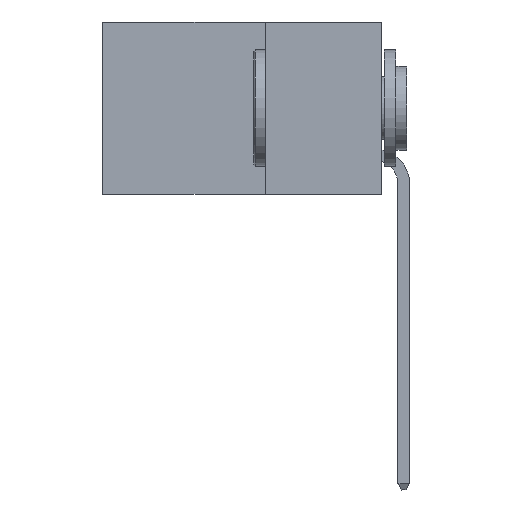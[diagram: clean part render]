
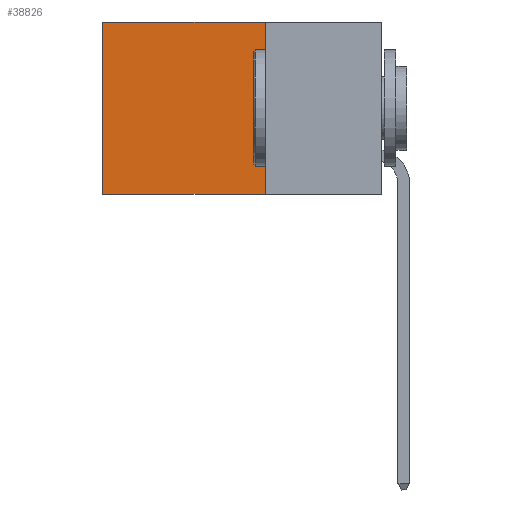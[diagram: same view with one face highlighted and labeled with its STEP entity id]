
A CAD part, left-side view. The second image highlights one B-rep face of the part: STEP entity #38826.
In plain terms, the highlighted planar face has unit normal (-1, 0, 0).
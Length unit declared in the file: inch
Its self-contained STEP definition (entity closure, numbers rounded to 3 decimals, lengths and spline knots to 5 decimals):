
#801 = LINE ( 'NONE', #12508, #32466 ) ;
#862 = LINE ( 'NONE', #8321, #16173 ) ;
#1087 = EDGE_CURVE ( 'NONE', #3247, #13767, #862, .T. ) ;
#1988 = EDGE_CURVE ( 'NONE', #23675, #22558, #22337, .T. ) ;
#3247 = VERTEX_POINT ( 'NONE', #31395 ) ;
#3289 = DIRECTION ( 'NONE',  ( 0., 0., -1. ) ) ;
#5727 = AXIS2_PLACEMENT_3D ( 'NONE', #35672, #17251, #38776 ) ;
#6565 = VECTOR ( 'NONE', #39519, 39.37008 ) ;
#8321 = CARTESIAN_POINT ( 'NONE',  ( 0.2875, 0.25, 0. ) ) ;
#8810 = CARTESIAN_POINT ( 'NONE',  ( 0.2875, 0.25, 0. ) ) ;
#12508 = CARTESIAN_POINT ( 'NONE',  ( 0.2875, 0.25, -0.37 ) ) ;
#13767 = VERTEX_POINT ( 'NONE', #15580 ) ;
#14165 = VECTOR ( 'NONE', #3289, 39.37008 ) ;
#14667 = ORIENTED_EDGE ( 'NONE', *, *, #1087, .F. ) ;
#15443 = CARTESIAN_POINT ( 'NONE',  ( 0.2875, 0.6, 0. ) ) ;
#15580 = CARTESIAN_POINT ( 'NONE',  ( 0.2875, 0.25, -0.37 ) ) ;
#15642 = LINE ( 'NONE', #8810, #6565 ) ;
#16173 = VECTOR ( 'NONE', #26666, 39.37008 ) ;
#17251 = DIRECTION ( 'NONE',  ( 1., 0., 0. ) ) ;
#19081 = CARTESIAN_POINT ( 'NONE',  ( 0.2875, 0.6, 0. ) ) ;
#19833 = ORIENTED_EDGE ( 'NONE', *, *, #1988, .T. ) ;
#19914 = EDGE_LOOP ( 'NONE', ( #19833, #32478, #14667, #32884 ) ) ;
#22337 = LINE ( 'NONE', #15443, #14165 ) ;
#22558 = VERTEX_POINT ( 'NONE', #24904 ) ;
#23013 = EDGE_CURVE ( 'NONE', #3247, #23675, #15642, .T. ) ;
#23189 = EDGE_CURVE ( 'NONE', #13767, #22558, #801, .T. ) ;
#23675 = VERTEX_POINT ( 'NONE', #19081 ) ;
#24904 = CARTESIAN_POINT ( 'NONE',  ( 0.2875, 0.6, -0.37 ) ) ;
#26666 = DIRECTION ( 'NONE',  ( 0., 0., -1. ) ) ;
#31193 = DIRECTION ( 'NONE',  ( 0., 1., 0. ) ) ;
#31395 = CARTESIAN_POINT ( 'NONE',  ( 0.2875, 0.25, 0. ) ) ;
#32466 = VECTOR ( 'NONE', #31193, 39.37008 ) ;
#32478 = ORIENTED_EDGE ( 'NONE', *, *, #23189, .F. ) ;
#32601 = PLANE ( 'NONE',  #5727 ) ;
#32884 = ORIENTED_EDGE ( 'NONE', *, *, #23013, .T. ) ;
#35565 = FACE_OUTER_BOUND ( 'NONE', #19914, .T. ) ;
#35672 = CARTESIAN_POINT ( 'NONE',  ( 0.2875, 0.25, 0. ) ) ;
#38776 = DIRECTION ( 'NONE',  ( 0., 0., -1. ) ) ;
#38826 = ADVANCED_FACE ( 'NONE', ( #35565 ), #32601, .F. ) ;
#39519 = DIRECTION ( 'NONE',  ( 0., 1., 0. ) ) ;
